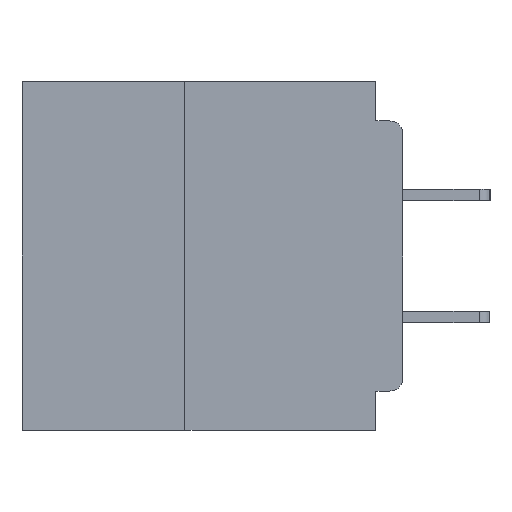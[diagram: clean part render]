
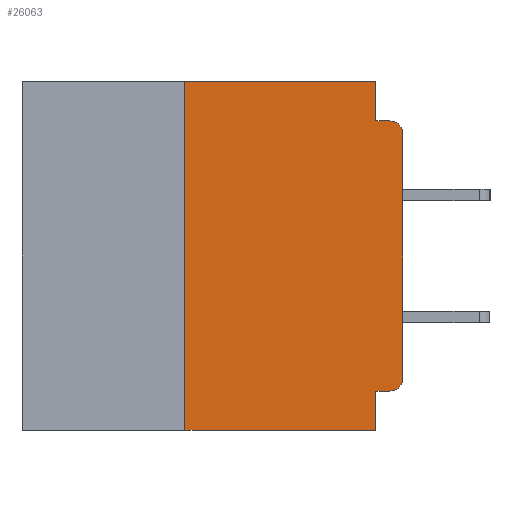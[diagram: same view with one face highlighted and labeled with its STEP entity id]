
A CAD part, left-side view. The second image highlights one B-rep face of the part: STEP entity #26063.
In plain terms, the highlighted planar face has unit normal (-1, 0, 0).
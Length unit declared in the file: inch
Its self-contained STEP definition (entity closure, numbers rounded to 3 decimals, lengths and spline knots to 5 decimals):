
#773 = CARTESIAN_POINT ( 'NONE',  ( 0., 0., -0.045 ) ) ;
#2799 = VERTEX_POINT ( 'NONE', #11708 ) ;
#3491 = DIRECTION ( 'NONE',  ( -1., 0., 0. ) ) ;
#4451 = ORIENTED_EDGE ( 'NONE', *, *, #5031, .F. ) ;
#5031 = EDGE_CURVE ( 'NONE', #36755, #2799, #45617, .T. ) ;
#7582 = LINE ( 'NONE', #13256, #35189 ) ;
#8201 = LINE ( 'NONE', #41402, #26235 ) ;
#8608 = VECTOR ( 'NONE', #17992, 39.37008 ) ;
#8701 = CIRCLE ( 'NONE', #11659, 0.015 ) ;
#8913 = CARTESIAN_POINT ( 'NONE',  ( 0., 0.015, -0.34 ) ) ;
#9584 = LINE ( 'NONE', #21067, #23219 ) ;
#10662 = ORIENTED_EDGE ( 'NONE', *, *, #37919, .T. ) ;
#11659 = AXIS2_PLACEMENT_3D ( 'NONE', #8913, #34097, #12512 ) ;
#11708 = CARTESIAN_POINT ( 'NONE',  ( 0., 0.031, -0.355 ) ) ;
#12028 = EDGE_CURVE ( 'NONE', #31341, #16698, #8201, .T. ) ;
#12512 = DIRECTION ( 'NONE',  ( 0., 0., -1. ) ) ;
#13062 = VECTOR ( 'NONE', #32249, 39.37008 ) ;
#13256 = CARTESIAN_POINT ( 'NONE',  ( 0., 0.031, 0. ) ) ;
#13961 = DIRECTION ( 'NONE',  ( 0., 0., 1. ) ) ;
#14281 = CARTESIAN_POINT ( 'NONE',  ( 0., 0.437, -0.4 ) ) ;
#14358 = CARTESIAN_POINT ( 'NONE',  ( 0., 0.031, -0.4 ) ) ;
#15274 = DIRECTION ( 'NONE',  ( 0., -1., 0. ) ) ;
#15284 = ORIENTED_EDGE ( 'NONE', *, *, #21265, .F. ) ;
#16432 = EDGE_CURVE ( 'NONE', #35821, #16834, #7582, .T. ) ;
#16456 = ORIENTED_EDGE ( 'NONE', *, *, #21991, .T. ) ;
#16632 = VECTOR ( 'NONE', #15274, 39.37008 ) ;
#16698 = VERTEX_POINT ( 'NONE', #29027 ) ;
#16834 = VERTEX_POINT ( 'NONE', #26183 ) ;
#17062 = VERTEX_POINT ( 'NONE', #38099 ) ;
#17992 = DIRECTION ( 'NONE',  ( 0., 0., -1. ) ) ;
#19212 = CARTESIAN_POINT ( 'NONE',  ( 0., 0.015, -0.355 ) ) ;
#19526 = CARTESIAN_POINT ( 'NONE',  ( 0., 0.437, 0. ) ) ;
#21067 = CARTESIAN_POINT ( 'NONE',  ( 0., 0., 0. ) ) ;
#21265 = EDGE_CURVE ( 'NONE', #16834, #28676, #27379, .T. ) ;
#21991 = EDGE_CURVE ( 'NONE', #36755, #45517, #8701, .T. ) ;
#22413 = CIRCLE ( 'NONE', #43767, 0.015 ) ;
#22571 = CARTESIAN_POINT ( 'NONE',  ( 0., 0.015, -0.045 ) ) ;
#22681 = LINE ( 'NONE', #14281, #13062 ) ;
#22884 = ORIENTED_EDGE ( 'NONE', *, *, #43020, .F. ) ;
#23017 = CARTESIAN_POINT ( 'NONE',  ( 0., 0., -0.34 ) ) ;
#23085 = DIRECTION ( 'NONE',  ( 0., 0., -1. ) ) ;
#23219 = VECTOR ( 'NONE', #13961, 39.37008 ) ;
#23909 = EDGE_CURVE ( 'NONE', #31341, #32146, #22681, .T. ) ;
#23996 = CARTESIAN_POINT ( 'NONE',  ( 0., 0.031, 0. ) ) ;
#24518 = ORIENTED_EDGE ( 'NONE', *, *, #12028, .F. ) ;
#24585 = ORIENTED_EDGE ( 'NONE', *, *, #26605, .T. ) ;
#25081 = CARTESIAN_POINT ( 'NONE',  ( 0., 0.015, -0.06 ) ) ;
#25890 = ORIENTED_EDGE ( 'NONE', *, *, #30944, .F. ) ;
#26063 = ADVANCED_FACE ( 'NONE', ( #36533 ), #37420, .F. ) ;
#26183 = CARTESIAN_POINT ( 'NONE',  ( 0., 0.031, -0.045 ) ) ;
#26235 = VECTOR ( 'NONE', #44993, 39.37008 ) ;
#26605 = EDGE_CURVE ( 'NONE', #17062, #28676, #22413, .T. ) ;
#27379 = LINE ( 'NONE', #773, #16632 ) ;
#27794 = LINE ( 'NONE', #14358, #8608 ) ;
#28676 = VERTEX_POINT ( 'NONE', #22571 ) ;
#28716 = DIRECTION ( 'NONE',  ( 0., 0., -1. ) ) ;
#29027 = CARTESIAN_POINT ( 'NONE',  ( 0., 0.25, 0. ) ) ;
#30391 = DIRECTION ( 'NONE',  ( 0., -1., 0. ) ) ;
#30944 = EDGE_CURVE ( 'NONE', #2799, #32146, #27794, .T. ) ;
#31341 = VERTEX_POINT ( 'NONE', #37943 ) ;
#32057 = EDGE_LOOP ( 'NONE', ( #10662, #24585, #15284, #45461, #22884, #24518, #36176, #25890, #4451, #16456 ) ) ;
#32146 = VERTEX_POINT ( 'NONE', #40492 ) ;
#32249 = DIRECTION ( 'NONE',  ( 0., -1., 0. ) ) ;
#34097 = DIRECTION ( 'NONE',  ( -1., 0., 0. ) ) ;
#35189 = VECTOR ( 'NONE', #38305, 39.37008 ) ;
#35821 = VERTEX_POINT ( 'NONE', #23996 ) ;
#35839 = CARTESIAN_POINT ( 'NONE',  ( 0., 0., -0.355 ) ) ;
#36105 = VECTOR ( 'NONE', #30391, 39.37008 ) ;
#36176 = ORIENTED_EDGE ( 'NONE', *, *, #23909, .T. ) ;
#36533 = FACE_OUTER_BOUND ( 'NONE', #32057, .T. ) ;
#36755 = VERTEX_POINT ( 'NONE', #19212 ) ;
#37420 = PLANE ( 'NONE',  #43148 ) ;
#37919 = EDGE_CURVE ( 'NONE', #45517, #17062, #9584, .T. ) ;
#37943 = CARTESIAN_POINT ( 'NONE',  ( 0., 0.25, -0.4 ) ) ;
#38099 = CARTESIAN_POINT ( 'NONE',  ( 0., 0., -0.06 ) ) ;
#38305 = DIRECTION ( 'NONE',  ( 0., 0., -1. ) ) ;
#38368 = VECTOR ( 'NONE', #39448, 39.37008 ) ;
#39448 = DIRECTION ( 'NONE',  ( 0., 1., 0. ) ) ;
#40492 = CARTESIAN_POINT ( 'NONE',  ( 0., 0.031, -0.4 ) ) ;
#40987 = CARTESIAN_POINT ( 'NONE',  ( 0., 0.437, 0. ) ) ;
#41402 = CARTESIAN_POINT ( 'NONE',  ( 0., 0.25, -0.4 ) ) ;
#43020 = EDGE_CURVE ( 'NONE', #16698, #35821, #45603, .T. ) ;
#43148 = AXIS2_PLACEMENT_3D ( 'NONE', #40987, #44598, #23085 ) ;
#43767 = AXIS2_PLACEMENT_3D ( 'NONE', #25081, #3491, #28716 ) ;
#44598 = DIRECTION ( 'NONE',  ( 1., 0., 0. ) ) ;
#44993 = DIRECTION ( 'NONE',  ( 0., 0., 1. ) ) ;
#45461 = ORIENTED_EDGE ( 'NONE', *, *, #16432, .F. ) ;
#45517 = VERTEX_POINT ( 'NONE', #23017 ) ;
#45603 = LINE ( 'NONE', #19526, #36105 ) ;
#45617 = LINE ( 'NONE', #35839, #38368 ) ;
